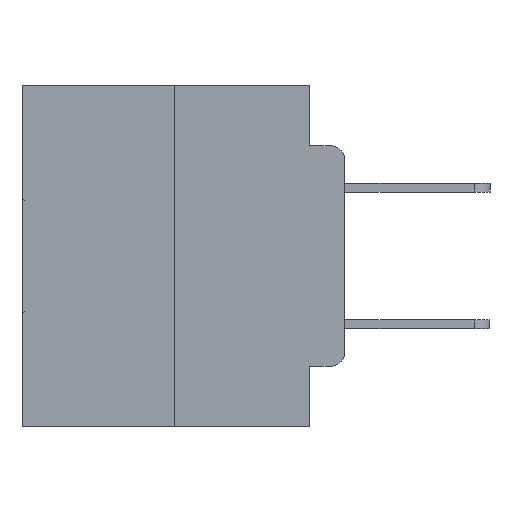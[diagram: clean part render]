
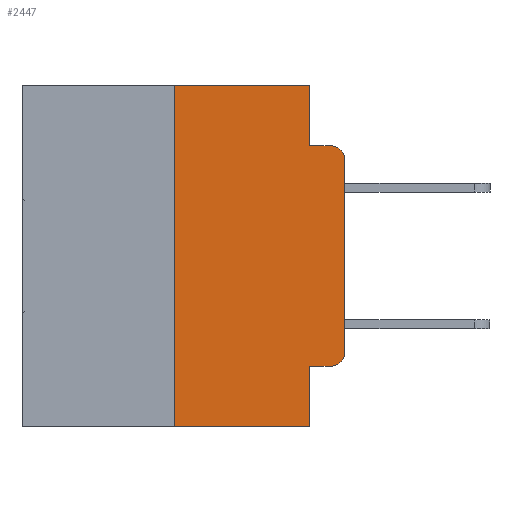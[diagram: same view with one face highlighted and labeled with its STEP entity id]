
A CAD part, left-side view. The second image highlights one B-rep face of the part: STEP entity #2447.
In plain terms, the highlighted planar face has unit normal (-1, 0, 0).
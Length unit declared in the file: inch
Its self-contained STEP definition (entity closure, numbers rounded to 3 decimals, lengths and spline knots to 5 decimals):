
#38 = CARTESIAN_POINT ( 'NONE',  ( 0., 0.051, 0. ) ) ;
#90 = CARTESIAN_POINT ( 'NONE',  ( 0., 0.473, 0. ) ) ;
#461 = CARTESIAN_POINT ( 'NONE',  ( 0., 0.051, -0.4115 ) ) ;
#546 = LINE ( 'NONE', #6536, #25433 ) ;
#1019 = CARTESIAN_POINT ( 'NONE',  ( 0., 0., 0. ) ) ;
#1123 = LINE ( 'NONE', #9171, #6047 ) ;
#1261 = ORIENTED_EDGE ( 'NONE', *, *, #23272, .T. ) ;
#1794 = LINE ( 'NONE', #461, #8231 ) ;
#1854 = CARTESIAN_POINT ( 'NONE',  ( 0., 0.02, -0.1085 ) ) ;
#2447 = ADVANCED_FACE ( 'NONE', ( #27557 ), #4841, .F. ) ;
#2722 = CARTESIAN_POINT ( 'NONE',  ( 0., 0.051, -0.0885 ) ) ;
#2878 = VECTOR ( 'NONE', #7357, 39.37008 ) ;
#3130 = VECTOR ( 'NONE', #3457, 39.37008 ) ;
#3406 = DIRECTION ( 'NONE',  ( -1., 0., 0. ) ) ;
#3457 = DIRECTION ( 'NONE',  ( 0., 0., 1. ) ) ;
#4276 = DIRECTION ( 'NONE',  ( 0., 0., -1. ) ) ;
#4281 = DIRECTION ( 'NONE',  ( 0., -1., 0. ) ) ;
#4841 = PLANE ( 'NONE',  #21207 ) ;
#5551 = VERTEX_POINT ( 'NONE', #11360 ) ;
#6047 = VECTOR ( 'NONE', #4281, 39.37008 ) ;
#6536 = CARTESIAN_POINT ( 'NONE',  ( 0., 0.25, 0. ) ) ;
#6644 = ORIENTED_EDGE ( 'NONE', *, *, #28688, .T. ) ;
#7088 = EDGE_CURVE ( 'NONE', #27591, #15329, #9327, .T. ) ;
#7357 = DIRECTION ( 'NONE',  ( 0., -1., 0. ) ) ;
#8231 = VECTOR ( 'NONE', #14990, 39.37008 ) ;
#8273 = VERTEX_POINT ( 'NONE', #28848 ) ;
#8741 = EDGE_CURVE ( 'NONE', #29234, #13979, #546, .T. ) ;
#9171 = CARTESIAN_POINT ( 'NONE',  ( 0., 0.473, -0.5 ) ) ;
#9325 = LINE ( 'NONE', #90, #2878 ) ;
#9327 = LINE ( 'NONE', #28921, #22923 ) ;
#9584 = LINE ( 'NONE', #1019, #3130 ) ;
#9730 = DIRECTION ( 'NONE',  ( 0., 0., -1. ) ) ;
#10045 = DIRECTION ( 'NONE',  ( 0., -1., 0. ) ) ;
#10371 = EDGE_CURVE ( 'NONE', #22443, #20188, #27221, .T. ) ;
#10725 = EDGE_LOOP ( 'NONE', ( #1261, #22818, #28815, #12666, #17988, #12699, #21759, #15018, #16532, #6644 ) ) ;
#11360 = CARTESIAN_POINT ( 'NONE',  ( 0., 0.02, -0.0885 ) ) ;
#11550 = DIRECTION ( 'NONE',  ( 0., 0., 1. ) ) ;
#12336 = CIRCLE ( 'NONE', #29602, 0.02 ) ;
#12666 = ORIENTED_EDGE ( 'NONE', *, *, #10371, .F. ) ;
#12699 = ORIENTED_EDGE ( 'NONE', *, *, #8741, .F. ) ;
#12752 = VERTEX_POINT ( 'NONE', #28662 ) ;
#13979 = VERTEX_POINT ( 'NONE', #30670 ) ;
#14578 = DIRECTION ( 'NONE',  ( 0., 0., -1. ) ) ;
#14990 = DIRECTION ( 'NONE',  ( 0., -1., 0. ) ) ;
#15018 = ORIENTED_EDGE ( 'NONE', *, *, #7088, .F. ) ;
#15280 = DIRECTION ( 'NONE',  ( 0., 0., -1. ) ) ;
#15329 = VERTEX_POINT ( 'NONE', #15872 ) ;
#15610 = AXIS2_PLACEMENT_3D ( 'NONE', #1854, #18785, #4276 ) ;
#15872 = CARTESIAN_POINT ( 'NONE',  ( 0., 0.051, -0.5 ) ) ;
#16532 = ORIENTED_EDGE ( 'NONE', *, *, #30298, .T. ) ;
#17071 = CARTESIAN_POINT ( 'NONE',  ( 0., 0., -0.3915 ) ) ;
#17935 = CARTESIAN_POINT ( 'NONE',  ( 0., 0.02, -0.3915 ) ) ;
#17988 = ORIENTED_EDGE ( 'NONE', *, *, #21306, .F. ) ;
#18031 = CIRCLE ( 'NONE', #15610, 0.02 ) ;
#18785 = DIRECTION ( 'NONE',  ( -1., 0., 0. ) ) ;
#19576 = VECTOR ( 'NONE', #10045, 39.37008 ) ;
#20065 = EDGE_CURVE ( 'NONE', #20188, #5551, #25906, .T. ) ;
#20188 = VERTEX_POINT ( 'NONE', #27263 ) ;
#20318 = DIRECTION ( 'NONE',  ( 0., 0., -1. ) ) ;
#21207 = AXIS2_PLACEMENT_3D ( 'NONE', #21737, #24145, #9730 ) ;
#21306 = EDGE_CURVE ( 'NONE', #13979, #22443, #9325, .T. ) ;
#21674 = EDGE_CURVE ( 'NONE', #12752, #5551, #18031, .T. ) ;
#21737 = CARTESIAN_POINT ( 'NONE',  ( 0., 0.473, 0. ) ) ;
#21759 = ORIENTED_EDGE ( 'NONE', *, *, #25269, .T. ) ;
#22443 = VERTEX_POINT ( 'NONE', #38 ) ;
#22487 = CARTESIAN_POINT ( 'NONE',  ( 0., 0.25, -0.5 ) ) ;
#22818 = ORIENTED_EDGE ( 'NONE', *, *, #21674, .T. ) ;
#22923 = VECTOR ( 'NONE', #14578, 39.37008 ) ;
#23272 = EDGE_CURVE ( 'NONE', #30860, #12752, #9584, .T. ) ;
#24145 = DIRECTION ( 'NONE',  ( 1., 0., 0. ) ) ;
#25269 = EDGE_CURVE ( 'NONE', #29234, #15329, #1123, .T. ) ;
#25433 = VECTOR ( 'NONE', #11550, 39.37008 ) ;
#25701 = VECTOR ( 'NONE', #15280, 39.37008 ) ;
#25906 = LINE ( 'NONE', #2722, #19576 ) ;
#27199 = CARTESIAN_POINT ( 'NONE',  ( 0., 0.051, 0. ) ) ;
#27221 = LINE ( 'NONE', #27199, #25701 ) ;
#27263 = CARTESIAN_POINT ( 'NONE',  ( 0., 0.051, -0.0885 ) ) ;
#27557 = FACE_OUTER_BOUND ( 'NONE', #10725, .T. ) ;
#27591 = VERTEX_POINT ( 'NONE', #28220 ) ;
#28220 = CARTESIAN_POINT ( 'NONE',  ( 0., 0.051, -0.4115 ) ) ;
#28662 = CARTESIAN_POINT ( 'NONE',  ( 0., 0., -0.1085 ) ) ;
#28688 = EDGE_CURVE ( 'NONE', #8273, #30860, #12336, .T. ) ;
#28815 = ORIENTED_EDGE ( 'NONE', *, *, #20065, .F. ) ;
#28848 = CARTESIAN_POINT ( 'NONE',  ( 0., 0.02, -0.4115 ) ) ;
#28921 = CARTESIAN_POINT ( 'NONE',  ( 0., 0.051, 0. ) ) ;
#29234 = VERTEX_POINT ( 'NONE', #22487 ) ;
#29602 = AXIS2_PLACEMENT_3D ( 'NONE', #17935, #3406, #20318 ) ;
#30298 = EDGE_CURVE ( 'NONE', #27591, #8273, #1794, .T. ) ;
#30670 = CARTESIAN_POINT ( 'NONE',  ( 0., 0.25, 0. ) ) ;
#30860 = VERTEX_POINT ( 'NONE', #17071 ) ;
